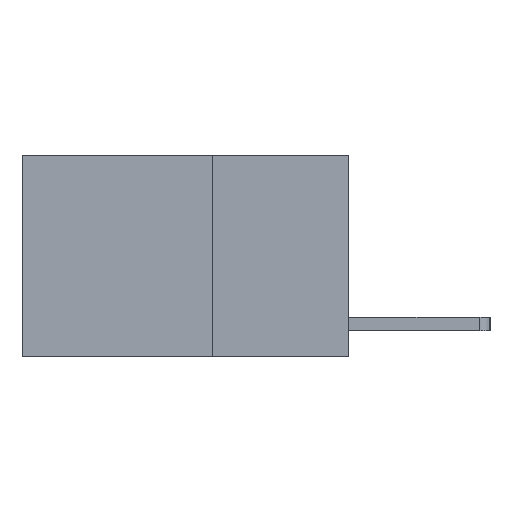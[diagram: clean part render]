
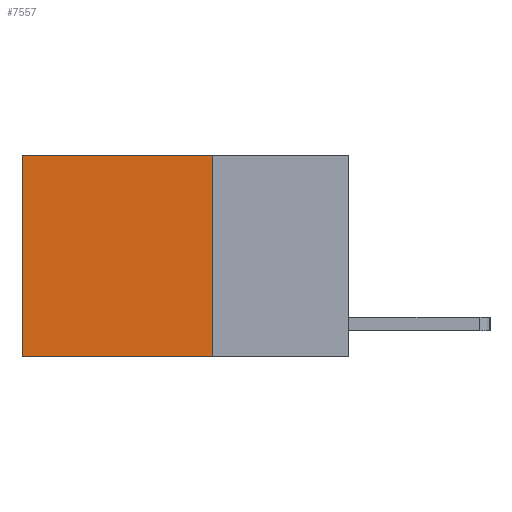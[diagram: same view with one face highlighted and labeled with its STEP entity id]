
A CAD part, left-side view. The second image highlights one B-rep face of the part: STEP entity #7557.
In plain terms, the highlighted planar face has unit normal (-1, 0, 0).
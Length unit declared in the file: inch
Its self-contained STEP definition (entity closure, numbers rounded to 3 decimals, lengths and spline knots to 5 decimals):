
#33 = DIRECTION ( 'NONE',  ( 0., 0., -1. ) ) ;
#82 = VERTEX_POINT ( 'NONE', #1712 ) ;
#87 = LINE ( 'NONE', #9527, #7012 ) ;
#153 = VERTEX_POINT ( 'NONE', #11652 ) ;
#572 = DIRECTION ( 'NONE',  ( 0., 0., -1. ) ) ;
#895 = PLANE ( 'NONE',  #1711 ) ;
#946 = CARTESIAN_POINT ( 'NONE',  ( 0.2625, 0.6, 0. ) ) ;
#1043 = CARTESIAN_POINT ( 'NONE',  ( 0.2625, 0.25, -0.37 ) ) ;
#1098 = VECTOR ( 'NONE', #10899, 39.37008 ) ;
#1131 = VECTOR ( 'NONE', #6668, 39.37008 ) ;
#1706 = ORIENTED_EDGE ( 'NONE', *, *, #1765, .T. ) ;
#1711 = AXIS2_PLACEMENT_3D ( 'NONE', #10737, #7223, #1827 ) ;
#1712 = CARTESIAN_POINT ( 'NONE',  ( 0.2625, 0.25, 0. ) ) ;
#1765 = EDGE_CURVE ( 'NONE', #82, #153, #8336, .T. ) ;
#1827 = DIRECTION ( 'NONE',  ( 0., 0., -1. ) ) ;
#2707 = EDGE_CURVE ( 'NONE', #153, #5083, #10108, .T. ) ;
#2976 = VECTOR ( 'NONE', #33, 39.37008 ) ;
#4687 = CARTESIAN_POINT ( 'NONE',  ( 0.2625, 0.25, -0.37 ) ) ;
#5083 = VERTEX_POINT ( 'NONE', #9605 ) ;
#5940 = LINE ( 'NONE', #4687, #1098 ) ;
#6668 = DIRECTION ( 'NONE',  ( 0., 1., 0. ) ) ;
#7012 = VECTOR ( 'NONE', #572, 39.37008 ) ;
#7046 = EDGE_LOOP ( 'NONE', ( #7848, #11098, #7235, #1706 ) ) ;
#7223 = DIRECTION ( 'NONE',  ( 1., 0., 0. ) ) ;
#7235 = ORIENTED_EDGE ( 'NONE', *, *, #11610, .F. ) ;
#7237 = FACE_OUTER_BOUND ( 'NONE', #7046, .T. ) ;
#7557 = ADVANCED_FACE ( 'NONE', ( #7237 ), #895, .F. ) ;
#7848 = ORIENTED_EDGE ( 'NONE', *, *, #2707, .T. ) ;
#8336 = LINE ( 'NONE', #10199, #1131 ) ;
#9527 = CARTESIAN_POINT ( 'NONE',  ( 0.2625, 0.25, 0. ) ) ;
#9605 = CARTESIAN_POINT ( 'NONE',  ( 0.2625, 0.6, -0.37 ) ) ;
#10108 = LINE ( 'NONE', #946, #2976 ) ;
#10199 = CARTESIAN_POINT ( 'NONE',  ( 0.2625, 0.25, 0. ) ) ;
#10737 = CARTESIAN_POINT ( 'NONE',  ( 0.2625, 0.25, 0. ) ) ;
#10772 = EDGE_CURVE ( 'NONE', #11324, #5083, #5940, .T. ) ;
#10899 = DIRECTION ( 'NONE',  ( 0., 1., 0. ) ) ;
#11098 = ORIENTED_EDGE ( 'NONE', *, *, #10772, .F. ) ;
#11324 = VERTEX_POINT ( 'NONE', #1043 ) ;
#11610 = EDGE_CURVE ( 'NONE', #82, #11324, #87, .T. ) ;
#11652 = CARTESIAN_POINT ( 'NONE',  ( 0.2625, 0.6, 0. ) ) ;
